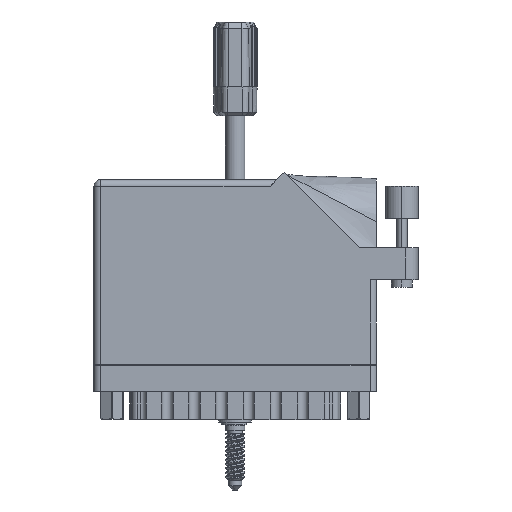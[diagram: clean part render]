
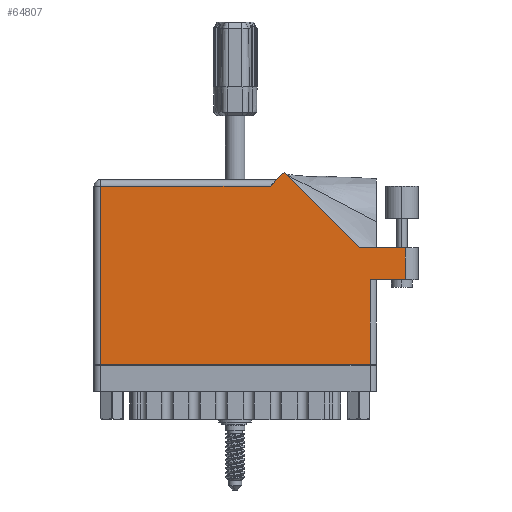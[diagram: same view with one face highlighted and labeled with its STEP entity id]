
A CAD part, front view. The second image highlights one B-rep face of the part: STEP entity #64807.
In plain terms, the highlighted face is planar.
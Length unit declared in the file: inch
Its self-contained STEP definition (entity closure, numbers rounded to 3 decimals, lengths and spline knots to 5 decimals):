
#1044 = VERTEX_POINT ( 'NONE', #73515 ) ;
#1871 = LINE ( 'NONE', #60484, #75097 ) ;
#2308 = VERTEX_POINT ( 'NONE', #3926 ) ;
#2348 = CARTESIAN_POINT ( 'NONE',  ( 2.656, 0.815, 0. ) ) ;
#3926 = CARTESIAN_POINT ( 'NONE',  ( 2.55242, 1.122, 0. ) ) ;
#4712 = ORIENTED_EDGE ( 'NONE', *, *, #62420, .T. ) ;
#4923 = LINE ( 'NONE', #79846, #87280 ) ;
#7505 = EDGE_CURVE ( 'NONE', #50111, #48865, #19101, .T. ) ;
#9500 = ORIENTED_EDGE ( 'NONE', *, *, #14334, .T. ) ;
#11814 = VECTOR ( 'NONE', #57829, 39.37008 ) ;
#11947 = ORIENTED_EDGE ( 'NONE', *, *, #57939, .T. ) ;
#14334 = EDGE_CURVE ( 'NONE', #29615, #2308, #24285, .T. ) ;
#15603 = EDGE_CURVE ( 'NONE', #2308, #69260, #52465, .T. ) ;
#16268 = AXIS2_PLACEMENT_3D ( 'NONE', #32802, #46974, #32477 ) ;
#18805 = VECTOR ( 'NONE', #46790, 39.37008 ) ;
#19101 = LINE ( 'NONE', #62203, #91328 ) ;
#22066 = LINE ( 'NONE', #66364, #25419 ) ;
#23459 = DIRECTION ( 'NONE',  ( -1., 0., 0. ) ) ;
#24285 = LINE ( 'NONE', #90352, #18805 ) ;
#25268 = CARTESIAN_POINT ( 'NONE',  ( 0.062, 0., 0. ) ) ;
#25419 = VECTOR ( 'NONE', #23459, 39.37008 ) ;
#25857 = VECTOR ( 'NONE', #66567, 39.37008 ) ;
#26511 = FACE_OUTER_BOUND ( 'NONE', #64508, .T. ) ;
#26822 = VERTEX_POINT ( 'NONE', #43776 ) ;
#27856 = CARTESIAN_POINT ( 'NONE',  ( 2.993, 1.122, 0. ) ) ;
#29615 = VERTEX_POINT ( 'NONE', #27856 ) ;
#32118 = DIRECTION ( 'NONE',  ( 1., 0., 0. ) ) ;
#32477 = DIRECTION ( 'NONE',  ( -1., 0., 0. ) ) ;
#32802 = CARTESIAN_POINT ( 'NONE',  ( 0., 1.775, 0. ) ) ;
#37805 = CARTESIAN_POINT ( 'NONE',  ( 1.82871, 1.84571, 0. ) ) ;
#39421 = EDGE_CURVE ( 'NONE', #69260, #58177, #81994, .T. ) ;
#40170 = ORIENTED_EDGE ( 'NONE', *, *, #51848, .T. ) ;
#40376 = CARTESIAN_POINT ( 'NONE',  ( 2.718, 0.815, 0. ) ) ;
#41682 = LINE ( 'NONE', #40376, #77715 ) ;
#43776 = CARTESIAN_POINT ( 'NONE',  ( 2.656, 0., 0. ) ) ;
#44335 = VERTEX_POINT ( 'NONE', #2348 ) ;
#45799 = VECTOR ( 'NONE', #90595, 39.37008 ) ;
#46790 = DIRECTION ( 'NONE',  ( -1., 0., 0. ) ) ;
#46974 = DIRECTION ( 'NONE',  ( 0., 0., -1. ) ) ;
#48865 = VERTEX_POINT ( 'NONE', #25268 ) ;
#50111 = VERTEX_POINT ( 'NONE', #60838 ) ;
#51826 = LINE ( 'NONE', #81100, #25857 ) ;
#51848 = EDGE_CURVE ( 'NONE', #58177, #50111, #22066, .T. ) ;
#52465 = LINE ( 'NONE', #85661, #11814 ) ;
#56236 = EDGE_CURVE ( 'NONE', #44335, #1044, #41682, .T. ) ;
#57829 = DIRECTION ( 'NONE',  ( -0.707, 0.707, 0. ) ) ;
#57939 = EDGE_CURVE ( 'NONE', #26822, #44335, #51826, .T. ) ;
#58177 = VERTEX_POINT ( 'NONE', #61800 ) ;
#60484 = CARTESIAN_POINT ( 'NONE',  ( 0., 0., 0. ) ) ;
#60558 = PLANE ( 'NONE',  #16268 ) ;
#60771 = EDGE_CURVE ( 'NONE', #48865, #26822, #1871, .T. ) ;
#60838 = CARTESIAN_POINT ( 'NONE',  ( 0.062, 1.713, 0. ) ) ;
#61800 = CARTESIAN_POINT ( 'NONE',  ( 1.696, 1.713, 0. ) ) ;
#62203 = CARTESIAN_POINT ( 'NONE',  ( 0.062, 0., 0. ) ) ;
#62420 = EDGE_CURVE ( 'NONE', #1044, #29615, #4923, .T. ) ;
#62471 = CARTESIAN_POINT ( 'NONE',  ( 1.758, 1.775, 0. ) ) ;
#64508 = EDGE_LOOP ( 'NONE', ( #71734, #4712, #9500, #84091, #65661, #40170, #67908, #88538, #11947 ) ) ;
#64807 = ADVANCED_FACE ( 'NONE', ( #26511 ), #60558, .F. ) ;
#65661 = ORIENTED_EDGE ( 'NONE', *, *, #39421, .T. ) ;
#66364 = CARTESIAN_POINT ( 'NONE',  ( 0., 1.713, 0. ) ) ;
#66567 = DIRECTION ( 'NONE',  ( 0., 1., 0. ) ) ;
#67908 = ORIENTED_EDGE ( 'NONE', *, *, #7505, .T. ) ;
#69260 = VERTEX_POINT ( 'NONE', #37805 ) ;
#71734 = ORIENTED_EDGE ( 'NONE', *, *, #56236, .T. ) ;
#73515 = CARTESIAN_POINT ( 'NONE',  ( 2.993, 0.815, 0. ) ) ;
#75097 = VECTOR ( 'NONE', #32118, 39.37008 ) ;
#75474 = DIRECTION ( 'NONE',  ( 0., -1., 0. ) ) ;
#77715 = VECTOR ( 'NONE', #92372, 39.37008 ) ;
#79846 = CARTESIAN_POINT ( 'NONE',  ( 2.993, 1.122, 0. ) ) ;
#81100 = CARTESIAN_POINT ( 'NONE',  ( 2.656, 0.815, 0. ) ) ;
#81994 = LINE ( 'NONE', #62471, #45799 ) ;
#84091 = ORIENTED_EDGE ( 'NONE', *, *, #15603, .T. ) ;
#85661 = CARTESIAN_POINT ( 'NONE',  ( 2.55242, 1.122, 0. ) ) ;
#87280 = VECTOR ( 'NONE', #93413, 39.37008 ) ;
#88538 = ORIENTED_EDGE ( 'NONE', *, *, #60771, .T. ) ;
#90352 = CARTESIAN_POINT ( 'NONE',  ( 3.118, 1.122, 0. ) ) ;
#90595 = DIRECTION ( 'NONE',  ( -0.707, -0.707, 0. ) ) ;
#91328 = VECTOR ( 'NONE', #75474, 39.37008 ) ;
#92372 = DIRECTION ( 'NONE',  ( 1., 0., 0. ) ) ;
#93413 = DIRECTION ( 'NONE',  ( 0., 1., 0. ) ) ;
